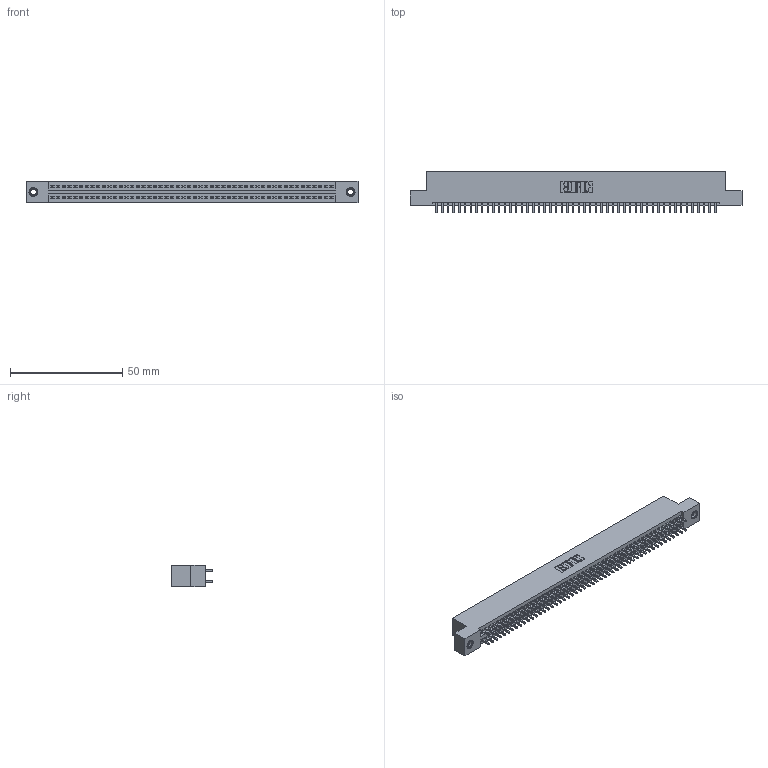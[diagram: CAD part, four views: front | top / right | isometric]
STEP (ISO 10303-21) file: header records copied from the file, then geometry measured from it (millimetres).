
FILE_DESCRIPTION (( 'STEP AP203' ), '1' );
FILE_NAME ('395-100-521-207.STEP', '2019-10-26T14:49:39', ( '' ), ( '' ), 'SwSTEP 2.0', 'SolidWorks 2016', '' );
FILE_SCHEMA (( 'CONFIG_CONTROL_DESIGN' ));
Length unit declared in the file: inch
Products named in the file (4): 345 Part_Flush Mounting Lugs - 0.156 Dia-TI; 345-292-001_345-293-121; 345-250-001_345-250-005-103; 395-100-521-207
Assembly tree (103 placements, depth 2):
  395-100-521-207
    345 Part_Flush Mounting Lugs - 0.156 Dia-TI
    345-292-001_345-293-121  x100
    345-250-001_345-250-005-103  x2
Bounding box: 148.21 x 18.72 x 9.4 mm (x, y, z)
Volume: 14417.1 mm3; surface area: 21228.1 mm2
Topology: 103 solids, 103 shells, 5186 faces, 15377 edges, 10110 vertices
Faces by surface type: plane 3412, cylinder 1758, cone 12, torus 4
Entity records: 39358 total; most frequent: CARTESIAN_POINT 6571, ORIENTED_EDGE 6498, DIRECTION 5811, EDGE_CURVE 3249, LINE 2897, VECTOR 2897, VERTEX_POINT 2160, AXIS2_PLACEMENT_3D 1457
